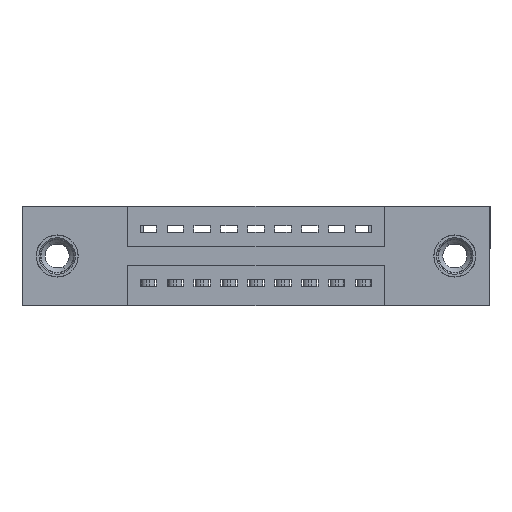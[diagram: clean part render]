
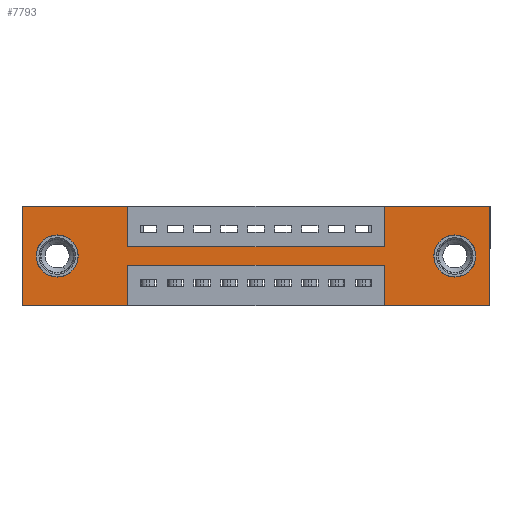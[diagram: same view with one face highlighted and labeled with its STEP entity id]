
A CAD part, front view. The second image highlights one B-rep face of the part: STEP entity #7793.
In plain terms, the highlighted planar face has unit normal (0, -1, 0).
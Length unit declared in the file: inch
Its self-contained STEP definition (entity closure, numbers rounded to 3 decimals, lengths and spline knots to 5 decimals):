
#112 = VERTEX_POINT ( 'NONE', #7168 ) ;
#145 = VERTEX_POINT ( 'NONE', #14646 ) ;
#151 = CIRCLE ( 'NONE', #6529, 0.078 ) ;
#298 = CARTESIAN_POINT ( 'NONE',  ( 0.13, 0., -0.185 ) ) ;
#505 = CARTESIAN_POINT ( 'NONE',  ( 0.3925, 0., 0. ) ) ;
#529 = DIRECTION ( 'NONE',  ( 0., 1., 0. ) ) ;
#623 = DIRECTION ( 'NONE',  ( 0., 0., -1. ) ) ;
#660 = CARTESIAN_POINT ( 'NONE',  ( 0.13, 0., -0.263 ) ) ;
#734 = VERTEX_POINT ( 'NONE', #1263 ) ;
#859 = VERTEX_POINT ( 'NONE', #6293 ) ;
#1025 = LINE ( 'NONE', #9160, #2394 ) ;
#1153 = CARTESIAN_POINT ( 'NONE',  ( 1.735, 0., -0.37 ) ) ;
#1231 = EDGE_CURVE ( 'NONE', #10415, #734, #3073, .T. ) ;
#1255 = ORIENTED_EDGE ( 'NONE', *, *, #6383, .F. ) ;
#1263 = CARTESIAN_POINT ( 'NONE',  ( 0., 0., -0.37 ) ) ;
#1468 = AXIS2_PLACEMENT_3D ( 'NONE', #1651, #529, #14006 ) ;
#1503 = VECTOR ( 'NONE', #6920, 39.37008 ) ;
#1651 = CARTESIAN_POINT ( 'NONE',  ( 1.605, 0., -0.185 ) ) ;
#1687 = VECTOR ( 'NONE', #7412, 39.37008 ) ;
#1738 = DIRECTION ( 'NONE',  ( 0., 1., 0. ) ) ;
#1760 = CARTESIAN_POINT ( 'NONE',  ( 0.3925, 0., -0.15 ) ) ;
#1765 = VECTOR ( 'NONE', #3356, 39.37008 ) ;
#1846 = VECTOR ( 'NONE', #4647, 39.37008 ) ;
#1917 = DIRECTION ( 'NONE',  ( 0., 0., 1. ) ) ;
#1980 = EDGE_CURVE ( 'NONE', #8006, #2517, #13431, .T. ) ;
#2180 = CARTESIAN_POINT ( 'NONE',  ( 0., 0., -0.37 ) ) ;
#2211 = ORIENTED_EDGE ( 'NONE', *, *, #11631, .T. ) ;
#2234 = ORIENTED_EDGE ( 'NONE', *, *, #11679, .T. ) ;
#2314 = EDGE_CURVE ( 'NONE', #145, #10637, #151, .T. ) ;
#2394 = VECTOR ( 'NONE', #7872, 39.37008 ) ;
#2464 = DIRECTION ( 'NONE',  ( -1., 0., 0. ) ) ;
#2517 = VERTEX_POINT ( 'NONE', #1153 ) ;
#2631 = CIRCLE ( 'NONE', #1468, 0.078 ) ;
#2732 = DIRECTION ( 'NONE',  ( 0., 1., 0. ) ) ;
#2990 = DIRECTION ( 'NONE',  ( 0., 0., -1. ) ) ;
#3011 = DIRECTION ( 'NONE',  ( 0., 0., -1. ) ) ;
#3041 = VERTEX_POINT ( 'NONE', #660 ) ;
#3073 = LINE ( 'NONE', #2180, #14018 ) ;
#3316 = CARTESIAN_POINT ( 'NONE',  ( 0.3925, 0., -0.37 ) ) ;
#3356 = DIRECTION ( 'NONE',  ( -1., 0., 0. ) ) ;
#3359 = CARTESIAN_POINT ( 'NONE',  ( 0., 0., 0. ) ) ;
#3413 = CARTESIAN_POINT ( 'NONE',  ( 0., 0., -0.37 ) ) ;
#3582 = EDGE_CURVE ( 'NONE', #12850, #8006, #15494, .T. ) ;
#3736 = AXIS2_PLACEMENT_3D ( 'NONE', #298, #2732, #3913 ) ;
#3908 = ORIENTED_EDGE ( 'NONE', *, *, #10505, .F. ) ;
#3913 = DIRECTION ( 'NONE',  ( 0., 0., 1. ) ) ;
#4024 = ORIENTED_EDGE ( 'NONE', *, *, #9722, .F. ) ;
#4241 = CARTESIAN_POINT ( 'NONE',  ( 0., 0., -0.37 ) ) ;
#4251 = CARTESIAN_POINT ( 'NONE',  ( 1.3425, 0., 0. ) ) ;
#4540 = CARTESIAN_POINT ( 'NONE',  ( 1.735, 0., 0. ) ) ;
#4647 = DIRECTION ( 'NONE',  ( 0., 0., 1. ) ) ;
#4739 = ORIENTED_EDGE ( 'NONE', *, *, #3582, .F. ) ;
#4776 = ORIENTED_EDGE ( 'NONE', *, *, #2314, .T. ) ;
#4839 = CARTESIAN_POINT ( 'NONE',  ( 1.735, 0., 0. ) ) ;
#5134 = DIRECTION ( 'NONE',  ( 1., 0., 0. ) ) ;
#5181 = DIRECTION ( 'NONE',  ( 1., 0., 0. ) ) ;
#5188 = VERTEX_POINT ( 'NONE', #1760 ) ;
#5432 = ORIENTED_EDGE ( 'NONE', *, *, #13377, .F. ) ;
#5530 = LINE ( 'NONE', #11634, #14772 ) ;
#5604 = VERTEX_POINT ( 'NONE', #11128 ) ;
#5697 = VECTOR ( 'NONE', #5134, 39.37008 ) ;
#6293 = CARTESIAN_POINT ( 'NONE',  ( 0.3925, 0., -0.22 ) ) ;
#6366 = LINE ( 'NONE', #3413, #1765 ) ;
#6383 = EDGE_CURVE ( 'NONE', #5604, #12850, #1025, .T. ) ;
#6407 = CARTESIAN_POINT ( 'NONE',  ( 1.3425, 0., -0.22 ) ) ;
#6416 = VECTOR ( 'NONE', #623, 39.37008 ) ;
#6529 = AXIS2_PLACEMENT_3D ( 'NONE', #11383, #1738, #2990 ) ;
#6587 = CARTESIAN_POINT ( 'NONE',  ( 0.3925, 0., -0.37 ) ) ;
#6766 = PLANE ( 'NONE',  #9957 ) ;
#6920 = DIRECTION ( 'NONE',  ( 0., 0., 1. ) ) ;
#6921 = DIRECTION ( 'NONE',  ( 0., -1., 0. ) ) ;
#7060 = LINE ( 'NONE', #3316, #13023 ) ;
#7168 = CARTESIAN_POINT ( 'NONE',  ( 0.13, 0., -0.107 ) ) ;
#7192 = EDGE_CURVE ( 'NONE', #2517, #14099, #6366, .T. ) ;
#7361 = ORIENTED_EDGE ( 'NONE', *, *, #1231, .F. ) ;
#7411 = CIRCLE ( 'NONE', #3736, 0.078 ) ;
#7412 = DIRECTION ( 'NONE',  ( 0., 0., -1. ) ) ;
#7509 = ORIENTED_EDGE ( 'NONE', *, *, #7192, .F. ) ;
#7569 = VERTEX_POINT ( 'NONE', #8763 ) ;
#7658 = ORIENTED_EDGE ( 'NONE', *, *, #12315, .F. ) ;
#7793 = ADVANCED_FACE ( 'NONE', ( #11319, #9968, #15207 ), #6766, .T. ) ;
#7872 = DIRECTION ( 'NONE',  ( 0., 0., 1. ) ) ;
#8006 = VERTEX_POINT ( 'NONE', #4839 ) ;
#8018 = EDGE_LOOP ( 'NONE', ( #8120, #10154, #8815, #7509, #11960, #4739, #1255, #4024, #7658, #5432, #3908, #7361 ) ) ;
#8120 = ORIENTED_EDGE ( 'NONE', *, *, #10166, .F. ) ;
#8172 = DIRECTION ( 'NONE',  ( 0., 1., 0. ) ) ;
#8389 = EDGE_LOOP ( 'NONE', ( #4776, #2211 ) ) ;
#8414 = ORIENTED_EDGE ( 'NONE', *, *, #10310, .T. ) ;
#8763 = CARTESIAN_POINT ( 'NONE',  ( 0., 0., 0. ) ) ;
#8815 = ORIENTED_EDGE ( 'NONE', *, *, #9086, .F. ) ;
#9086 = EDGE_CURVE ( 'NONE', #14099, #14382, #13634, .T. ) ;
#9160 = CARTESIAN_POINT ( 'NONE',  ( 1.3425, 0., 0. ) ) ;
#9250 = CARTESIAN_POINT ( 'NONE',  ( 0.13, 0., -0.185 ) ) ;
#9456 = CARTESIAN_POINT ( 'NONE',  ( 1.3425, 0., -0.37 ) ) ;
#9722 = EDGE_CURVE ( 'NONE', #5188, #5604, #5530, .T. ) ;
#9957 = AXIS2_PLACEMENT_3D ( 'NONE', #4241, #6921, #3011 ) ;
#9968 = FACE_BOUND ( 'NONE', #14562, .T. ) ;
#10008 = CARTESIAN_POINT ( 'NONE',  ( 0., 0., 0. ) ) ;
#10154 = ORIENTED_EDGE ( 'NONE', *, *, #12010, .F. ) ;
#10166 = EDGE_CURVE ( 'NONE', #859, #10415, #7060, .T. ) ;
#10240 = LINE ( 'NONE', #11070, #15097 ) ;
#10310 = EDGE_CURVE ( 'NONE', #3041, #112, #7411, .T. ) ;
#10415 = VERTEX_POINT ( 'NONE', #6587 ) ;
#10505 = EDGE_CURVE ( 'NONE', #734, #7569, #13954, .T. ) ;
#10637 = VERTEX_POINT ( 'NONE', #10736 ) ;
#10687 = VERTEX_POINT ( 'NONE', #11551 ) ;
#10706 = DIRECTION ( 'NONE',  ( 0., 0., -1. ) ) ;
#10736 = CARTESIAN_POINT ( 'NONE',  ( 1.605, 0., -0.263 ) ) ;
#11070 = CARTESIAN_POINT ( 'NONE',  ( 0.3925, 0., -0.22 ) ) ;
#11128 = CARTESIAN_POINT ( 'NONE',  ( 1.3425, 0., -0.15 ) ) ;
#11222 = CIRCLE ( 'NONE', #12776, 0.078 ) ;
#11319 = FACE_BOUND ( 'NONE', #8389, .T. ) ;
#11383 = CARTESIAN_POINT ( 'NONE',  ( 1.605, 0., -0.185 ) ) ;
#11551 = CARTESIAN_POINT ( 'NONE',  ( 0.3925, 0., 0. ) ) ;
#11631 = EDGE_CURVE ( 'NONE', #10637, #145, #2631, .T. ) ;
#11634 = CARTESIAN_POINT ( 'NONE',  ( 0.3925, 0., -0.15 ) ) ;
#11679 = EDGE_CURVE ( 'NONE', #112, #3041, #11222, .T. ) ;
#11960 = ORIENTED_EDGE ( 'NONE', *, *, #1980, .F. ) ;
#12010 = EDGE_CURVE ( 'NONE', #14382, #859, #10240, .T. ) ;
#12315 = EDGE_CURVE ( 'NONE', #10687, #5188, #15470, .T. ) ;
#12653 = CARTESIAN_POINT ( 'NONE',  ( 0., 0., 0. ) ) ;
#12724 = DIRECTION ( 'NONE',  ( 1., 0., 0. ) ) ;
#12776 = AXIS2_PLACEMENT_3D ( 'NONE', #9250, #8172, #1917 ) ;
#12850 = VERTEX_POINT ( 'NONE', #4251 ) ;
#13023 = VECTOR ( 'NONE', #10706, 39.37008 ) ;
#13377 = EDGE_CURVE ( 'NONE', #7569, #10687, #14275, .T. ) ;
#13431 = LINE ( 'NONE', #4540, #1687 ) ;
#13634 = LINE ( 'NONE', #14287, #1503 ) ;
#13954 = LINE ( 'NONE', #3359, #1846 ) ;
#14006 = DIRECTION ( 'NONE',  ( 0., 0., -1. ) ) ;
#14018 = VECTOR ( 'NONE', #14362, 39.37008 ) ;
#14099 = VERTEX_POINT ( 'NONE', #9456 ) ;
#14275 = LINE ( 'NONE', #12653, #14677 ) ;
#14287 = CARTESIAN_POINT ( 'NONE',  ( 1.3425, 0., -0.37 ) ) ;
#14362 = DIRECTION ( 'NONE',  ( -1., 0., 0. ) ) ;
#14382 = VERTEX_POINT ( 'NONE', #6407 ) ;
#14562 = EDGE_LOOP ( 'NONE', ( #2234, #8414 ) ) ;
#14646 = CARTESIAN_POINT ( 'NONE',  ( 1.605, 0., -0.107 ) ) ;
#14677 = VECTOR ( 'NONE', #5181, 39.37008 ) ;
#14772 = VECTOR ( 'NONE', #12724, 39.37008 ) ;
#15097 = VECTOR ( 'NONE', #2464, 39.37008 ) ;
#15207 = FACE_OUTER_BOUND ( 'NONE', #8018, .T. ) ;
#15470 = LINE ( 'NONE', #505, #6416 ) ;
#15494 = LINE ( 'NONE', #10008, #5697 ) ;
